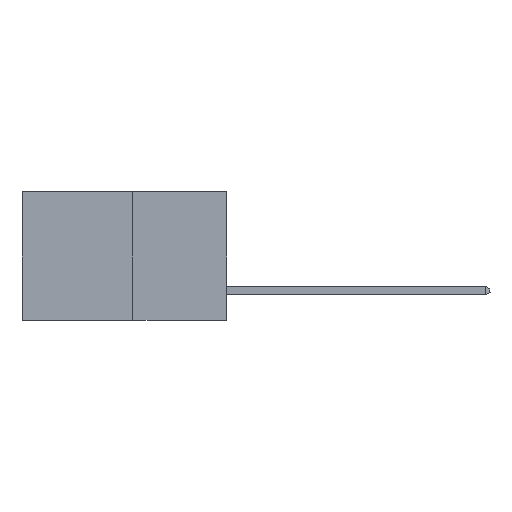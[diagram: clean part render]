
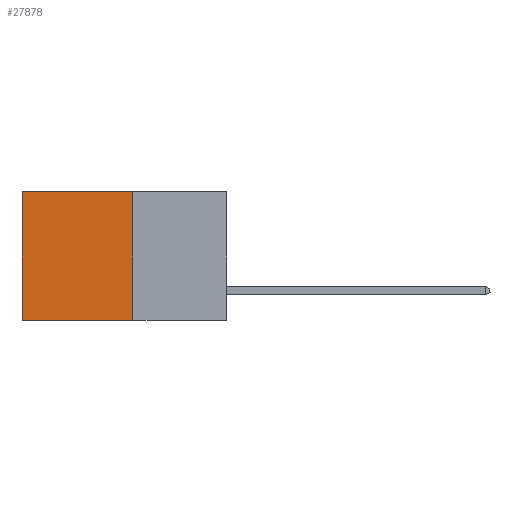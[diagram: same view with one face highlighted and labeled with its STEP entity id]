
A CAD part, left-side view. The second image highlights one B-rep face of the part: STEP entity #27878.
In plain terms, the highlighted planar face has unit normal (-1, 0, 0).
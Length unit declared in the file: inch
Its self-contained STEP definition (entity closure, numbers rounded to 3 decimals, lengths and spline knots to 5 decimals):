
#342 = DIRECTION ( 'NONE',  ( 0., 0., -1. ) ) ;
#840 = CARTESIAN_POINT ( 'NONE',  ( 0.277, 0.59, -0.37 ) ) ;
#1652 = AXIS2_PLACEMENT_3D ( 'NONE', #11435, #13628, #342 ) ;
#1776 = DIRECTION ( 'NONE',  ( 0., 1., 0. ) ) ;
#2147 = EDGE_CURVE ( 'NONE', #16396, #23155, #14576, .T. ) ;
#2391 = PLANE ( 'NONE',  #1652 ) ;
#2399 = ORIENTED_EDGE ( 'NONE', *, *, #21656, .F. ) ;
#2809 = VECTOR ( 'NONE', #19881, 39.37008 ) ;
#3658 = FACE_OUTER_BOUND ( 'NONE', #7275, .T. ) ;
#4584 = DIRECTION ( 'NONE',  ( 0., 0., -1. ) ) ;
#6018 = VECTOR ( 'NONE', #16641, 39.37008 ) ;
#7275 = EDGE_LOOP ( 'NONE', ( #27400, #17992, #2399, #7436 ) ) ;
#7374 = VECTOR ( 'NONE', #4584, 39.37008 ) ;
#7436 = ORIENTED_EDGE ( 'NONE', *, *, #2147, .T. ) ;
#7638 = VERTEX_POINT ( 'NONE', #19443 ) ;
#8496 = CARTESIAN_POINT ( 'NONE',  ( 0.277, 0.27, -0.37 ) ) ;
#9317 = VERTEX_POINT ( 'NONE', #840 ) ;
#10131 = CARTESIAN_POINT ( 'NONE',  ( 0.277, 0.27, -0.37 ) ) ;
#11233 = LINE ( 'NONE', #10131, #6018 ) ;
#11435 = CARTESIAN_POINT ( 'NONE',  ( 0.277, 0.27, -0.37 ) ) ;
#11719 = VECTOR ( 'NONE', #1776, 39.37008 ) ;
#12413 = LINE ( 'NONE', #8496, #11719 ) ;
#13275 = LINE ( 'NONE', #24158, #7374 ) ;
#13628 = DIRECTION ( 'NONE',  ( 1., 0., 0. ) ) ;
#14576 = LINE ( 'NONE', #20005, #2809 ) ;
#14967 = CARTESIAN_POINT ( 'NONE',  ( 0.277, 0.59, 0. ) ) ;
#16272 = CARTESIAN_POINT ( 'NONE',  ( 0.277, 0.27, 0. ) ) ;
#16396 = VERTEX_POINT ( 'NONE', #16272 ) ;
#16641 = DIRECTION ( 'NONE',  ( 0., 0., -1. ) ) ;
#17992 = ORIENTED_EDGE ( 'NONE', *, *, #25937, .F. ) ;
#19443 = CARTESIAN_POINT ( 'NONE',  ( 0.277, 0.27, -0.37 ) ) ;
#19881 = DIRECTION ( 'NONE',  ( 0., 1., 0. ) ) ;
#20005 = CARTESIAN_POINT ( 'NONE',  ( 0.277, 0.27, 0. ) ) ;
#21656 = EDGE_CURVE ( 'NONE', #16396, #7638, #11233, .T. ) ;
#21994 = EDGE_CURVE ( 'NONE', #23155, #9317, #13275, .T. ) ;
#23155 = VERTEX_POINT ( 'NONE', #14967 ) ;
#24158 = CARTESIAN_POINT ( 'NONE',  ( 0.277, 0.59, -0.37 ) ) ;
#25937 = EDGE_CURVE ( 'NONE', #7638, #9317, #12413, .T. ) ;
#27400 = ORIENTED_EDGE ( 'NONE', *, *, #21994, .T. ) ;
#27878 = ADVANCED_FACE ( 'NONE', ( #3658 ), #2391, .F. ) ;
